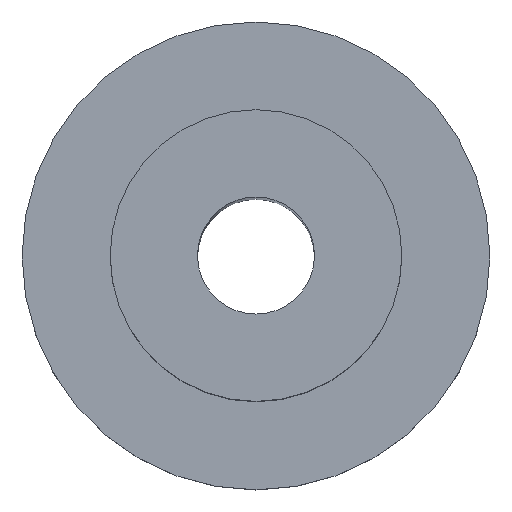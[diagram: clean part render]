
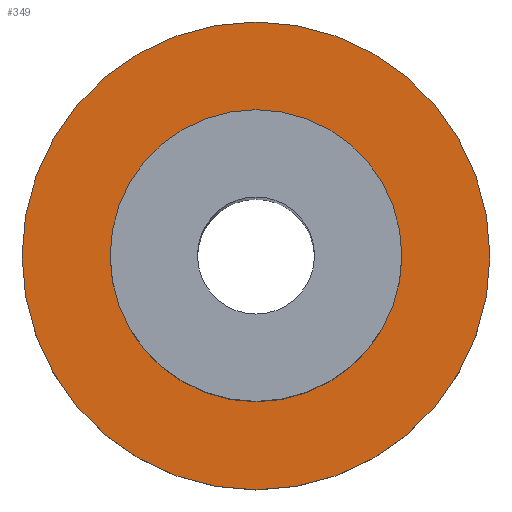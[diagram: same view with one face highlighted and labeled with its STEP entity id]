
A CAD part, top view. The second image highlights one B-rep face of the part: STEP entity #349.
In plain terms, the highlighted planar face has unit normal (0, 0, 1).
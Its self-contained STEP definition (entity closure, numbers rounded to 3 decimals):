
#14 = CARTESIAN_POINT ( 'NONE',  ( 2.438, 0., -3.937 ) ) ;
#20 = DIRECTION ( 'NONE',  ( 1., 0., 0. ) ) ;
#23 = DIRECTION ( 'NONE',  ( 0., 0., 1. ) ) ;
#24 = CARTESIAN_POINT ( 'NONE',  ( 0., 0., -3.937 ) ) ;
#26 = CARTESIAN_POINT ( 'NONE',  ( -2.438, 0., -3.937 ) ) ;
#35 = AXIS2_PLACEMENT_3D ( 'NONE', #24, #23, #20 ) ;
#53 = AXIS2_PLACEMENT_3D ( 'NONE', #106, #105, #103 ) ;
#60 = AXIS2_PLACEMENT_3D ( 'NONE', #200, #201, #185 ) ;
#89 = CIRCLE ( 'NONE', #35, 3.912 ) ;
#99 = CARTESIAN_POINT ( 'NONE',  ( 3.912, 0., -3.937 ) ) ;
#102 = AXIS2_PLACEMENT_3D ( 'NONE', #293, #292, #286 ) ;
#103 = DIRECTION ( 'NONE',  ( 1., 0., 0. ) ) ;
#105 = DIRECTION ( 'NONE',  ( 0., 0., 1. ) ) ;
#106 = CARTESIAN_POINT ( 'NONE',  ( 0., 0., -3.937 ) ) ;
#126 = ORIENTED_EDGE ( 'NONE', *, *, #318, .T. ) ;
#138 = CIRCLE ( 'NONE', #53, 2.438 ) ;
#147 = AXIS2_PLACEMENT_3D ( 'NONE', #324, #302, #301 ) ;
#154 = FACE_OUTER_BOUND ( 'NONE', #352, .T. ) ;
#165 = FACE_BOUND ( 'NONE', #325, .T. ) ;
#171 = CARTESIAN_POINT ( 'NONE',  ( -3.912, 0., -3.937 ) ) ;
#183 = CIRCLE ( 'NONE', #147, 3.912 ) ;
#184 = VERTEX_POINT ( 'NONE', #26 ) ;
#185 = DIRECTION ( 'NONE',  ( -1., 0., 0. ) ) ;
#191 = CIRCLE ( 'NONE', #102, 2.438 ) ;
#192 = VERTEX_POINT ( 'NONE', #171 ) ;
#194 = PLANE ( 'NONE',  #60 ) ;
#200 = CARTESIAN_POINT ( 'NONE',  ( 0., 2.438, -3.937 ) ) ;
#201 = DIRECTION ( 'NONE',  ( 0., 0., -1. ) ) ;
#286 = DIRECTION ( 'NONE',  ( 1., 0., 0. ) ) ;
#292 = DIRECTION ( 'NONE',  ( 0., 0., 1. ) ) ;
#293 = CARTESIAN_POINT ( 'NONE',  ( 0., 0., -3.937 ) ) ;
#296 = VERTEX_POINT ( 'NONE', #14 ) ;
#301 = DIRECTION ( 'NONE',  ( 1., 0., 0. ) ) ;
#302 = DIRECTION ( 'NONE',  ( 0., 0., 1. ) ) ;
#318 = EDGE_CURVE ( 'NONE', #381, #192, #183, .T. ) ;
#320 = EDGE_CURVE ( 'NONE', #296, #184, #191, .T. ) ;
#324 = CARTESIAN_POINT ( 'NONE',  ( 0., 0., -3.937 ) ) ;
#325 = EDGE_LOOP ( 'NONE', ( #375, #380 ) ) ;
#349 = ADVANCED_FACE ( 'NONE', ( #165, #154 ), #194, .F. ) ;
#352 = EDGE_LOOP ( 'NONE', ( #126, #416 ) ) ;
#374 = EDGE_CURVE ( 'NONE', #184, #296, #138, .T. ) ;
#375 = ORIENTED_EDGE ( 'NONE', *, *, #320, .F. ) ;
#380 = ORIENTED_EDGE ( 'NONE', *, *, #374, .F. ) ;
#381 = VERTEX_POINT ( 'NONE', #99 ) ;
#416 = ORIENTED_EDGE ( 'NONE', *, *, #417, .T. ) ;
#417 = EDGE_CURVE ( 'NONE', #192, #381, #89, .T. ) ;
